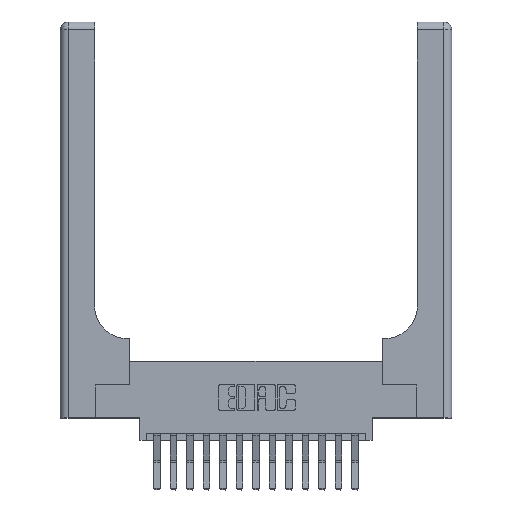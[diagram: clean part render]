
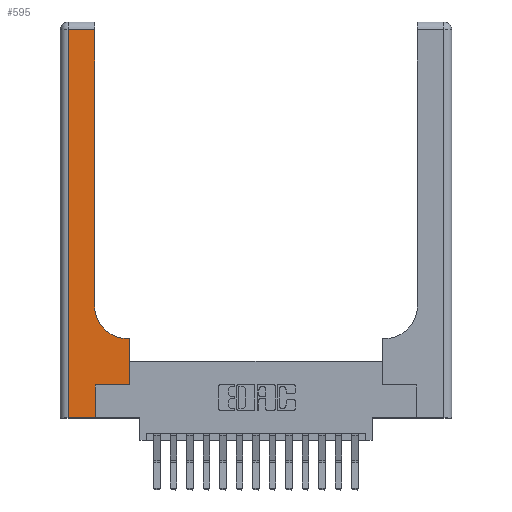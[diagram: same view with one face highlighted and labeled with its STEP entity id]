
A CAD part, top view. The second image highlights one B-rep face of the part: STEP entity #595.
In plain terms, the highlighted planar face has unit normal (0, 0, 1).
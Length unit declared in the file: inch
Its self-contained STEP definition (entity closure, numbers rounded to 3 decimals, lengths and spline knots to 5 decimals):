
#27 = ORIENTED_EDGE ( 'NONE', *, *, #5823, .T. ) ;
#188 = ORIENTED_EDGE ( 'NONE', *, *, #8419, .T. ) ;
#517 = EDGE_CURVE ( 'NONE', #5524, #14716, #6250, .T. ) ;
#524 = LINE ( 'NONE', #17399, #8397 ) ;
#595 = ADVANCED_FACE ( 'NONE', ( #15015 ), #947, .F. ) ;
#772 = CARTESIAN_POINT ( 'NONE',  ( 0.26, 0.6, 0.37 ) ) ;
#916 = DIRECTION ( 'NONE',  ( 0., 1., 0. ) ) ;
#939 = CARTESIAN_POINT ( 'NONE',  ( 0.06, 3., 0.37 ) ) ;
#947 = PLANE ( 'NONE',  #16634 ) ;
#1188 = CARTESIAN_POINT ( 'NONE',  ( 0.26, 3., 0.37 ) ) ;
#1908 = VERTEX_POINT ( 'NONE', #4164 ) ;
#2059 = CARTESIAN_POINT ( 'NONE',  ( 0., 2.94, 0.37 ) ) ;
#2331 = CARTESIAN_POINT ( 'NONE',  ( 0., 3., 0.37 ) ) ;
#2345 = CARTESIAN_POINT ( 'NONE',  ( 0.528, 0.6, 0.37 ) ) ;
#2363 = DIRECTION ( 'NONE',  ( 1., 0., 0. ) ) ;
#2405 = CARTESIAN_POINT ( 'NONE',  ( 0.51, 0.6, 0.37 ) ) ;
#2672 = ORIENTED_EDGE ( 'NONE', *, *, #6813, .T. ) ;
#2959 = CARTESIAN_POINT ( 'NONE',  ( 0.06, 0., 0.37 ) ) ;
#3187 = EDGE_CURVE ( 'NONE', #12964, #10652, #524, .T. ) ;
#3810 = DIRECTION ( 'NONE',  ( 0., 0., -1. ) ) ;
#3956 = EDGE_LOOP ( 'NONE', ( #16852, #7227, #27, #11881, #5484, #2672, #188, #12286, #17299 ) ) ;
#4103 = CARTESIAN_POINT ( 'NONE',  ( 0.528, 0.25, 0.37 ) ) ;
#4164 = CARTESIAN_POINT ( 'NONE',  ( 0.06, 2.94, 0.37 ) ) ;
#4794 = DIRECTION ( 'NONE',  ( 0., 1., 0. ) ) ;
#5321 = VECTOR ( 'NONE', #6722, 39.37008 ) ;
#5484 = ORIENTED_EDGE ( 'NONE', *, *, #3187, .T. ) ;
#5524 = VERTEX_POINT ( 'NONE', #2345 ) ;
#5708 = LINE ( 'NONE', #16661, #17237 ) ;
#5823 = EDGE_CURVE ( 'NONE', #1908, #7309, #17791, .T. ) ;
#6250 = LINE ( 'NONE', #772, #17494 ) ;
#6288 = CARTESIAN_POINT ( 'NONE',  ( 0.26, 2.94, 0.37 ) ) ;
#6448 = VECTOR ( 'NONE', #14170, 39.37008 ) ;
#6706 = DIRECTION ( 'NONE',  ( 0., 0., -1. ) ) ;
#6722 = DIRECTION ( 'NONE',  ( -1., 0., 0. ) ) ;
#6742 = CARTESIAN_POINT ( 'NONE',  ( 0., 0., 0.37 ) ) ;
#6813 = EDGE_CURVE ( 'NONE', #10652, #14718, #5708, .T. ) ;
#7068 = EDGE_CURVE ( 'NONE', #14716, #7210, #7417, .T. ) ;
#7199 = CARTESIAN_POINT ( 'NONE',  ( 0.265, 0.25, 0.37 ) ) ;
#7210 = VERTEX_POINT ( 'NONE', #10152 ) ;
#7227 = ORIENTED_EDGE ( 'NONE', *, *, #12265, .T. ) ;
#7309 = VERTEX_POINT ( 'NONE', #2959 ) ;
#7417 = CIRCLE ( 'NONE', #13871, 0.25 ) ;
#7810 = VECTOR ( 'NONE', #916, 39.37008 ) ;
#7840 = DIRECTION ( 'NONE',  ( 0., -1., 0. ) ) ;
#8026 = CARTESIAN_POINT ( 'NONE',  ( 0.265, 0., 0.37 ) ) ;
#8140 = LINE ( 'NONE', #6742, #12092 ) ;
#8397 = VECTOR ( 'NONE', #4794, 39.37008 ) ;
#8419 = EDGE_CURVE ( 'NONE', #14718, #5524, #15479, .T. ) ;
#9133 = DIRECTION ( 'NONE',  ( 1., 0., 0. ) ) ;
#9707 = DIRECTION ( 'NONE',  ( -1., 0., 0. ) ) ;
#10152 = CARTESIAN_POINT ( 'NONE',  ( 0.26, 0.85, 0.37 ) ) ;
#10544 = DIRECTION ( 'NONE',  ( -1., 0., 0. ) ) ;
#10631 = EDGE_CURVE ( 'NONE', #7309, #12964, #8140, .T. ) ;
#10652 = VERTEX_POINT ( 'NONE', #7199 ) ;
#11881 = ORIENTED_EDGE ( 'NONE', *, *, #10631, .T. ) ;
#12092 = VECTOR ( 'NONE', #2363, 39.37008 ) ;
#12221 = CARTESIAN_POINT ( 'NONE',  ( 0.528, 0.25, 0.37 ) ) ;
#12265 = EDGE_CURVE ( 'NONE', #17321, #1908, #14841, .T. ) ;
#12286 = ORIENTED_EDGE ( 'NONE', *, *, #517, .T. ) ;
#12964 = VERTEX_POINT ( 'NONE', #8026 ) ;
#13585 = LINE ( 'NONE', #1188, #7810 ) ;
#13871 = AXIS2_PLACEMENT_3D ( 'NONE', #14927, #6706, #9133 ) ;
#14170 = DIRECTION ( 'NONE',  ( 0., 1., 0. ) ) ;
#14716 = VERTEX_POINT ( 'NONE', #2405 ) ;
#14718 = VERTEX_POINT ( 'NONE', #12221 ) ;
#14841 = LINE ( 'NONE', #2059, #5321 ) ;
#14927 = CARTESIAN_POINT ( 'NONE',  ( 0.51, 0.85, 0.37 ) ) ;
#15015 = FACE_OUTER_BOUND ( 'NONE', #3956, .T. ) ;
#15187 = VECTOR ( 'NONE', #7840, 39.37008 ) ;
#15479 = LINE ( 'NONE', #4103, #6448 ) ;
#16634 = AXIS2_PLACEMENT_3D ( 'NONE', #2331, #3810, #9707 ) ;
#16661 = CARTESIAN_POINT ( 'NONE',  ( 0.265, 0.25, 0.37 ) ) ;
#16852 = ORIENTED_EDGE ( 'NONE', *, *, #18132, .T. ) ;
#17237 = VECTOR ( 'NONE', #18180, 39.37008 ) ;
#17299 = ORIENTED_EDGE ( 'NONE', *, *, #7068, .T. ) ;
#17321 = VERTEX_POINT ( 'NONE', #6288 ) ;
#17399 = CARTESIAN_POINT ( 'NONE',  ( 0.265, 0., 0.37 ) ) ;
#17494 = VECTOR ( 'NONE', #10544, 39.37008 ) ;
#17791 = LINE ( 'NONE', #939, #15187 ) ;
#18132 = EDGE_CURVE ( 'NONE', #7210, #17321, #13585, .T. ) ;
#18180 = DIRECTION ( 'NONE',  ( 1., 0., 0. ) ) ;
